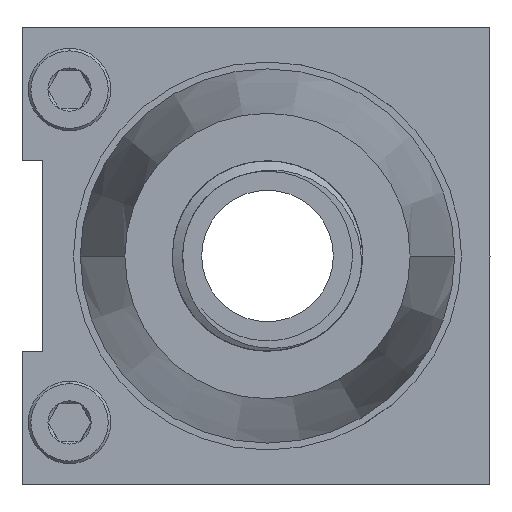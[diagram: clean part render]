
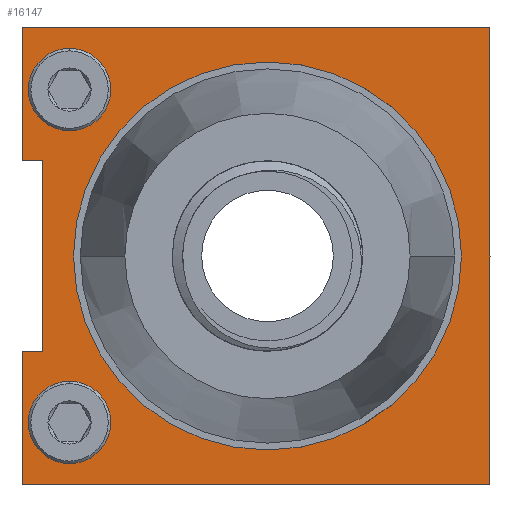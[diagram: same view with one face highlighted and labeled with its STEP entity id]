
A CAD part, left-side view. The second image highlights one B-rep face of the part: STEP entity #16147.
In plain terms, the highlighted face is planar.
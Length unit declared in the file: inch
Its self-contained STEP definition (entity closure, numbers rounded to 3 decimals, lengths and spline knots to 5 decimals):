
#506 = CARTESIAN_POINT ( 'NONE',  ( 1.0375, -0.125, 0. ) ) ;
#512 = VERTEX_POINT ( 'NONE', #23634 ) ;
#601 = CARTESIAN_POINT ( 'NONE',  ( 0., -1.23, 0. ) ) ;
#730 = EDGE_CURVE ( 'NONE', #7004, #10284, #21023, .T. ) ;
#761 = CIRCLE ( 'NONE', #9839, 0.06693 ) ;
#1268 = CARTESIAN_POINT ( 'NONE',  ( 0.22943, -0.125, 0. ) ) ;
#1342 = DIRECTION ( 'NONE',  ( 0., 0., 1. ) ) ;
#1405 = CARTESIAN_POINT ( 'NONE',  ( 0.1625, -0.125, 0. ) ) ;
#1503 = CARTESIAN_POINT ( 'NONE',  ( 0.35, -0.055, 0. ) ) ;
#1518 = LINE ( 'NONE', #16581, #10938 ) ;
#1527 = CARTESIAN_POINT ( 'NONE',  ( 0.1625, -0.125, 0. ) ) ;
#1648 = ORIENTED_EDGE ( 'NONE', *, *, #24470, .T. ) ;
#1650 = VERTEX_POINT ( 'NONE', #21948 ) ;
#1706 = FACE_OUTER_BOUND ( 'NONE', #23417, .T. ) ;
#1765 = EDGE_CURVE ( 'NONE', #9788, #10184, #7044, .T. ) ;
#1916 = CARTESIAN_POINT ( 'NONE',  ( 1.0375, -0.125, 0. ) ) ;
#2147 = ORIENTED_EDGE ( 'NONE', *, *, #18431, .T. ) ;
#2585 = FACE_BOUND ( 'NONE', #5547, .T. ) ;
#2718 = CARTESIAN_POINT ( 'NONE',  ( 0.85, 0., 0. ) ) ;
#3201 = CARTESIAN_POINT ( 'NONE',  ( 0.6, -0.6454, 0. ) ) ;
#3347 = AXIS2_PLACEMENT_3D ( 'NONE', #506, #3978, #8042 ) ;
#3564 = PLANE ( 'NONE',  #3692 ) ;
#3608 = EDGE_CURVE ( 'NONE', #16593, #13458, #761, .T. ) ;
#3660 = CARTESIAN_POINT ( 'NONE',  ( 0.97057, -0.125, 0. ) ) ;
#3692 = AXIS2_PLACEMENT_3D ( 'NONE', #5296, #1342, #8994 ) ;
#3978 = DIRECTION ( 'NONE',  ( 0., 0., 1. ) ) ;
#4048 = EDGE_CURVE ( 'NONE', #10984, #12105, #7896, .T. ) ;
#4080 = VECTOR ( 'NONE', #4705, 39.37008 ) ;
#4081 = DIRECTION ( 'NONE',  ( -1., 0., 0. ) ) ;
#4705 = DIRECTION ( 'NONE',  ( -1., 0., 0. ) ) ;
#5130 = ORIENTED_EDGE ( 'NONE', *, *, #730, .F. ) ;
#5296 = CARTESIAN_POINT ( 'NONE',  ( 0., 0., 0. ) ) ;
#5366 = ORIENTED_EDGE ( 'NONE', *, *, #3608, .T. ) ;
#5537 = CARTESIAN_POINT ( 'NONE',  ( 1.2, -1.23, 0. ) ) ;
#5547 = EDGE_LOOP ( 'NONE', ( #1648, #19370 ) ) ;
#5728 = CIRCLE ( 'NONE', #3347, 0.06693 ) ;
#5855 = LINE ( 'NONE', #18945, #14543 ) ;
#5984 = DIRECTION ( 'NONE',  ( 0., 1., 0. ) ) ;
#6071 = EDGE_CURVE ( 'NONE', #10284, #23633, #5855, .T. ) ;
#6175 = CARTESIAN_POINT ( 'NONE',  ( 0., 0., 0. ) ) ;
#6347 = ORIENTED_EDGE ( 'NONE', *, *, #4048, .F. ) ;
#6799 = VECTOR ( 'NONE', #15242, 39.37008 ) ;
#6829 = VECTOR ( 'NONE', #13029, 39.37008 ) ;
#6898 = DIRECTION ( 'NONE',  ( 1., 0., 0. ) ) ;
#7004 = VERTEX_POINT ( 'NONE', #14045 ) ;
#7044 = CIRCLE ( 'NONE', #20067, 0.06693 ) ;
#7085 = DIRECTION ( 'NONE',  ( 1., 0., 0. ) ) ;
#7479 = DIRECTION ( 'NONE',  ( 1., 0., 0. ) ) ;
#7862 = CARTESIAN_POINT ( 'NONE',  ( 0.35, 0., 0. ) ) ;
#7896 = LINE ( 'NONE', #6175, #9401 ) ;
#8042 = DIRECTION ( 'NONE',  ( 1., 0., 0. ) ) ;
#8381 = ORIENTED_EDGE ( 'NONE', *, *, #13080, .F. ) ;
#8396 = CARTESIAN_POINT ( 'NONE',  ( 0.85, -0.055, 0. ) ) ;
#8820 = LINE ( 'NONE', #22071, #4080 ) ;
#8880 = CIRCLE ( 'NONE', #9265, 0.51 ) ;
#8994 = DIRECTION ( 'NONE',  ( 1., 0., 0. ) ) ;
#9084 = ORIENTED_EDGE ( 'NONE', *, *, #19618, .T. ) ;
#9239 = FACE_BOUND ( 'NONE', #19612, .T. ) ;
#9265 = AXIS2_PLACEMENT_3D ( 'NONE', #14581, #15065, #12846 ) ;
#9401 = VECTOR ( 'NONE', #22994, 39.37008 ) ;
#9444 = DIRECTION ( 'NONE',  ( 0., 1., 0. ) ) ;
#9571 = CARTESIAN_POINT ( 'NONE',  ( 0.85, 0., 0. ) ) ;
#9788 = VERTEX_POINT ( 'NONE', #23789 ) ;
#9803 = LINE ( 'NONE', #19198, #10436 ) ;
#9839 = AXIS2_PLACEMENT_3D ( 'NONE', #1916, #24410, #7479 ) ;
#10184 = VERTEX_POINT ( 'NONE', #1268 ) ;
#10284 = VERTEX_POINT ( 'NONE', #1503 ) ;
#10436 = VECTOR ( 'NONE', #5984, 39.37008 ) ;
#10793 = DIRECTION ( 'NONE',  ( 1., 0., 0. ) ) ;
#10938 = VECTOR ( 'NONE', #10793, 39.37008 ) ;
#10984 = VERTEX_POINT ( 'NONE', #17458 ) ;
#12072 = ORIENTED_EDGE ( 'NONE', *, *, #15195, .F. ) ;
#12105 = VERTEX_POINT ( 'NONE', #2718 ) ;
#12846 = DIRECTION ( 'NONE',  ( 1., 0., 0. ) ) ;
#13029 = DIRECTION ( 'NONE',  ( 0., -1., 0. ) ) ;
#13080 = EDGE_CURVE ( 'NONE', #12105, #7004, #20589, .T. ) ;
#13101 = VERTEX_POINT ( 'NONE', #20705 ) ;
#13244 = DIRECTION ( 'NONE',  ( 1., 0., 0. ) ) ;
#13458 = VERTEX_POINT ( 'NONE', #16423 ) ;
#14045 = CARTESIAN_POINT ( 'NONE',  ( 0.85, -0.055, 0. ) ) ;
#14424 = DIRECTION ( 'NONE',  ( 0., 0., 1. ) ) ;
#14543 = VECTOR ( 'NONE', #9444, 39.37008 ) ;
#14581 = CARTESIAN_POINT ( 'NONE',  ( 0.6, -0.6454, 0. ) ) ;
#15065 = DIRECTION ( 'NONE',  ( 0., 0., 1. ) ) ;
#15195 = EDGE_CURVE ( 'NONE', #1650, #20038, #16729, .T. ) ;
#15197 = ORIENTED_EDGE ( 'NONE', *, *, #6071, .F. ) ;
#15242 = DIRECTION ( 'NONE',  ( 0., -1., 0. ) ) ;
#15781 = EDGE_LOOP ( 'NONE', ( #2147, #23452 ) ) ;
#16147 = ADVANCED_FACE ( 'NONE', ( #17535, #2585, #9239, #1706 ), #3564, .F. ) ;
#16222 = DIRECTION ( 'NONE',  ( 0., 0., 1. ) ) ;
#16423 = CARTESIAN_POINT ( 'NONE',  ( 1.10443, -0.125, 0. ) ) ;
#16581 = CARTESIAN_POINT ( 'NONE',  ( 0., -1.23, 0. ) ) ;
#16587 = DIRECTION ( 'NONE',  ( 0., 0., 1. ) ) ;
#16593 = VERTEX_POINT ( 'NONE', #3660 ) ;
#16729 = LINE ( 'NONE', #19074, #6829 ) ;
#16847 = AXIS2_PLACEMENT_3D ( 'NONE', #1527, #16587, #13244 ) ;
#16899 = EDGE_CURVE ( 'NONE', #23633, #1650, #8820, .T. ) ;
#17458 = CARTESIAN_POINT ( 'NONE',  ( 1.2, 0., 0. ) ) ;
#17535 = FACE_BOUND ( 'NONE', #15781, .T. ) ;
#18036 = ORIENTED_EDGE ( 'NONE', *, *, #22977, .F. ) ;
#18362 = VERTEX_POINT ( 'NONE', #5537 ) ;
#18431 = EDGE_CURVE ( 'NONE', #13101, #512, #19520, .T. ) ;
#18522 = EDGE_CURVE ( 'NONE', #18362, #10984, #9803, .T. ) ;
#18945 = CARTESIAN_POINT ( 'NONE',  ( 0.35, 0., 0. ) ) ;
#19074 = CARTESIAN_POINT ( 'NONE',  ( 0., 0., 0. ) ) ;
#19198 = CARTESIAN_POINT ( 'NONE',  ( 1.2, 0., 0. ) ) ;
#19370 = ORIENTED_EDGE ( 'NONE', *, *, #1765, .T. ) ;
#19426 = ORIENTED_EDGE ( 'NONE', *, *, #16899, .F. ) ;
#19520 = CIRCLE ( 'NONE', #24234, 0.51 ) ;
#19612 = EDGE_LOOP ( 'NONE', ( #9084, #5366 ) ) ;
#19618 = EDGE_CURVE ( 'NONE', #13458, #16593, #5728, .T. ) ;
#19654 = VECTOR ( 'NONE', #4081, 39.37008 ) ;
#19931 = EDGE_CURVE ( 'NONE', #512, #13101, #8880, .T. ) ;
#20038 = VERTEX_POINT ( 'NONE', #601 ) ;
#20067 = AXIS2_PLACEMENT_3D ( 'NONE', #1405, #16222, #7085 ) ;
#20408 = CIRCLE ( 'NONE', #16847, 0.06693 ) ;
#20589 = LINE ( 'NONE', #9571, #6799 ) ;
#20705 = CARTESIAN_POINT ( 'NONE',  ( 1.11, -0.6454, 0. ) ) ;
#21023 = LINE ( 'NONE', #8396, #19654 ) ;
#21049 = ORIENTED_EDGE ( 'NONE', *, *, #18522, .F. ) ;
#21948 = CARTESIAN_POINT ( 'NONE',  ( 0., 0., 0. ) ) ;
#22071 = CARTESIAN_POINT ( 'NONE',  ( 0., 0., 0. ) ) ;
#22977 = EDGE_CURVE ( 'NONE', #20038, #18362, #1518, .T. ) ;
#22994 = DIRECTION ( 'NONE',  ( -1., 0., 0. ) ) ;
#23417 = EDGE_LOOP ( 'NONE', ( #5130, #8381, #6347, #21049, #18036, #12072, #19426, #15197 ) ) ;
#23452 = ORIENTED_EDGE ( 'NONE', *, *, #19931, .T. ) ;
#23633 = VERTEX_POINT ( 'NONE', #7862 ) ;
#23634 = CARTESIAN_POINT ( 'NONE',  ( 0.09, -0.6454, 0. ) ) ;
#23789 = CARTESIAN_POINT ( 'NONE',  ( 0.09557, -0.125, 0. ) ) ;
#24234 = AXIS2_PLACEMENT_3D ( 'NONE', #3201, #14424, #6898 ) ;
#24410 = DIRECTION ( 'NONE',  ( 0., 0., 1. ) ) ;
#24470 = EDGE_CURVE ( 'NONE', #10184, #9788, #20408, .T. ) ;
